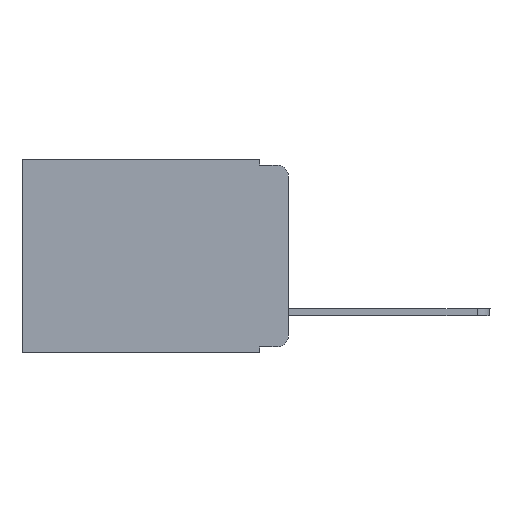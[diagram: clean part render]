
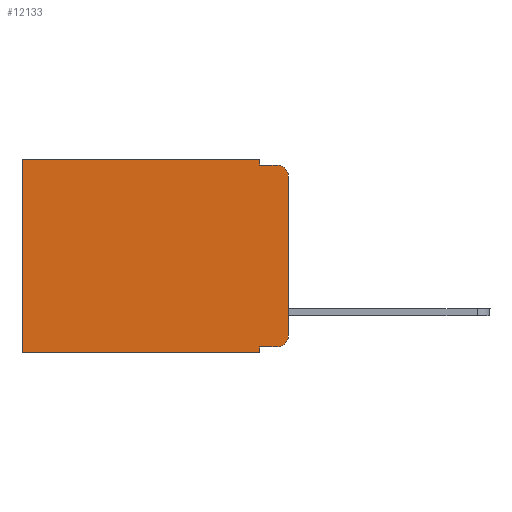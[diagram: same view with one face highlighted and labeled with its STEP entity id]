
A CAD part, left-side view. The second image highlights one B-rep face of the part: STEP entity #12133.
In plain terms, the highlighted planar face has unit normal (-1, 0, 0).
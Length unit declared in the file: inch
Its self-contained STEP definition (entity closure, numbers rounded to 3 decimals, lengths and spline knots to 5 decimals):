
#79 = LINE ( 'NONE', #8217, #16747 ) ;
#538 = EDGE_CURVE ( 'NONE', #7096, #14317, #5625, .T. ) ;
#716 = EDGE_CURVE ( 'NONE', #10554, #12443, #3504, .T. ) ;
#820 = EDGE_CURVE ( 'NONE', #14317, #1258, #17788, .T. ) ;
#956 = DIRECTION ( 'NONE',  ( 1., 0., 0. ) ) ;
#1258 = VERTEX_POINT ( 'NONE', #5561 ) ;
#1425 = ORIENTED_EDGE ( 'NONE', *, *, #17079, .T. ) ;
#1522 = ORIENTED_EDGE ( 'NONE', *, *, #14105, .F. ) ;
#1708 = LINE ( 'NONE', #3079, #5700 ) ;
#1888 = LINE ( 'NONE', #14687, #5671 ) ;
#2331 = FACE_OUTER_BOUND ( 'NONE', #16522, .T. ) ;
#2385 = CARTESIAN_POINT ( 'NONE',  ( 0.298, 0.02, -0.333 ) ) ;
#2732 = CARTESIAN_POINT ( 'NONE',  ( 0.298, 0.051, -0.01 ) ) ;
#3079 = CARTESIAN_POINT ( 'NONE',  ( 0.298, 0.473, 0. ) ) ;
#3271 = VECTOR ( 'NONE', #10160, 39.37008 ) ;
#3504 = LINE ( 'NONE', #14479, #14113 ) ;
#3517 = CARTESIAN_POINT ( 'NONE',  ( 0.298, 0.051, -0.343 ) ) ;
#3606 = CARTESIAN_POINT ( 'NONE',  ( 0.298, 0., 0. ) ) ;
#4181 = VERTEX_POINT ( 'NONE', #14793 ) ;
#4260 = CARTESIAN_POINT ( 'NONE',  ( 0.298, 0.02, -0.03 ) ) ;
#4449 = CARTESIAN_POINT ( 'NONE',  ( 0.298, 0.051, -0.333 ) ) ;
#4819 = LINE ( 'NONE', #5098, #10898 ) ;
#5098 = CARTESIAN_POINT ( 'NONE',  ( 0.298, 0., -0.343 ) ) ;
#5561 = CARTESIAN_POINT ( 'NONE',  ( 0.298, 0., -0.313 ) ) ;
#5593 = EDGE_CURVE ( 'NONE', #6025, #12443, #18056, .T. ) ;
#5611 = ORIENTED_EDGE ( 'NONE', *, *, #13543, .F. ) ;
#5625 = LINE ( 'NONE', #6999, #10276 ) ;
#5671 = VECTOR ( 'NONE', #6098, 39.37008 ) ;
#5700 = VECTOR ( 'NONE', #17080, 39.37008 ) ;
#6025 = VERTEX_POINT ( 'NONE', #11012 ) ;
#6098 = DIRECTION ( 'NONE',  ( 0., 0., -1. ) ) ;
#6179 = DIRECTION ( 'NONE',  ( 0., 1., 0. ) ) ;
#6212 = ORIENTED_EDGE ( 'NONE', *, *, #10836, .F. ) ;
#6289 = ORIENTED_EDGE ( 'NONE', *, *, #820, .T. ) ;
#6838 = DIRECTION ( 'NONE',  ( 0., 0., -1. ) ) ;
#6999 = CARTESIAN_POINT ( 'NONE',  ( 0.298, 0.051, -0.333 ) ) ;
#7096 = VERTEX_POINT ( 'NONE', #4449 ) ;
#7510 = CARTESIAN_POINT ( 'NONE',  ( 0.298, 0.051, 0. ) ) ;
#7910 = PLANE ( 'NONE',  #12261 ) ;
#8217 = CARTESIAN_POINT ( 'NONE',  ( 0.298, 0., 0. ) ) ;
#8429 = EDGE_CURVE ( 'NONE', #6025, #1258, #1888, .T. ) ;
#8469 = DIRECTION ( 'NONE',  ( -1., 0., 0. ) ) ;
#8696 = LINE ( 'NONE', #7510, #3271 ) ;
#9204 = DIRECTION ( 'NONE',  ( 0., 1., 0. ) ) ;
#9370 = DIRECTION ( 'NONE',  ( 0., 0., -1. ) ) ;
#9481 = LINE ( 'NONE', #15244, #13765 ) ;
#10160 = DIRECTION ( 'NONE',  ( 0., 0., -1. ) ) ;
#10276 = VECTOR ( 'NONE', #11190, 39.37008 ) ;
#10531 = EDGE_CURVE ( 'NONE', #14591, #11901, #79, .T. ) ;
#10554 = VERTEX_POINT ( 'NONE', #2732 ) ;
#10811 = CARTESIAN_POINT ( 'NONE',  ( 0.298, 0.473, 0. ) ) ;
#10836 = EDGE_CURVE ( 'NONE', #12099, #4181, #4819, .T. ) ;
#10898 = VECTOR ( 'NONE', #9204, 39.37008 ) ;
#11012 = CARTESIAN_POINT ( 'NONE',  ( 0.298, 0., -0.03 ) ) ;
#11089 = ORIENTED_EDGE ( 'NONE', *, *, #10531, .T. ) ;
#11149 = CARTESIAN_POINT ( 'NONE',  ( 0.298, 0.02, -0.313 ) ) ;
#11190 = DIRECTION ( 'NONE',  ( 0., -1., 0. ) ) ;
#11339 = ORIENTED_EDGE ( 'NONE', *, *, #716, .F. ) ;
#11643 = DIRECTION ( 'NONE',  ( 0., -1., 0. ) ) ;
#11901 = VERTEX_POINT ( 'NONE', #10811 ) ;
#12099 = VERTEX_POINT ( 'NONE', #3517 ) ;
#12133 = ADVANCED_FACE ( 'NONE', ( #2331 ), #7910, .F. ) ;
#12261 = AXIS2_PLACEMENT_3D ( 'NONE', #3606, #956, #9370 ) ;
#12436 = DIRECTION ( 'NONE',  ( 0., 0., -1. ) ) ;
#12443 = VERTEX_POINT ( 'NONE', #13012 ) ;
#12914 = ORIENTED_EDGE ( 'NONE', *, *, #8429, .F. ) ;
#13012 = CARTESIAN_POINT ( 'NONE',  ( 0.298, 0.02, -0.01 ) ) ;
#13543 = EDGE_CURVE ( 'NONE', #14591, #10554, #9481, .T. ) ;
#13765 = VECTOR ( 'NONE', #17830, 39.37008 ) ;
#14105 = EDGE_CURVE ( 'NONE', #7096, #12099, #8696, .T. ) ;
#14113 = VECTOR ( 'NONE', #11643, 39.37008 ) ;
#14317 = VERTEX_POINT ( 'NONE', #2385 ) ;
#14439 = CARTESIAN_POINT ( 'NONE',  ( 0.298, 0.051, 0. ) ) ;
#14479 = CARTESIAN_POINT ( 'NONE',  ( 0.298, 0.051, -0.01 ) ) ;
#14591 = VERTEX_POINT ( 'NONE', #14439 ) ;
#14687 = CARTESIAN_POINT ( 'NONE',  ( 0.298, 0., 0. ) ) ;
#14793 = CARTESIAN_POINT ( 'NONE',  ( 0.298, 0.473, -0.343 ) ) ;
#15121 = AXIS2_PLACEMENT_3D ( 'NONE', #4260, #8469, #6838 ) ;
#15244 = CARTESIAN_POINT ( 'NONE',  ( 0.298, 0.051, 0. ) ) ;
#15434 = AXIS2_PLACEMENT_3D ( 'NONE', #11149, #16559, #12436 ) ;
#16277 = ORIENTED_EDGE ( 'NONE', *, *, #5593, .T. ) ;
#16522 = EDGE_LOOP ( 'NONE', ( #12914, #16277, #11339, #5611, #11089, #1425, #6212, #1522, #17388, #6289 ) ) ;
#16559 = DIRECTION ( 'NONE',  ( -1., 0., 0. ) ) ;
#16747 = VECTOR ( 'NONE', #6179, 39.37008 ) ;
#17079 = EDGE_CURVE ( 'NONE', #11901, #4181, #1708, .T. ) ;
#17080 = DIRECTION ( 'NONE',  ( 0., 0., -1. ) ) ;
#17388 = ORIENTED_EDGE ( 'NONE', *, *, #538, .T. ) ;
#17788 = CIRCLE ( 'NONE', #15434, 0.02 ) ;
#17830 = DIRECTION ( 'NONE',  ( 0., 0., -1. ) ) ;
#18056 = CIRCLE ( 'NONE', #15121, 0.02 ) ;
